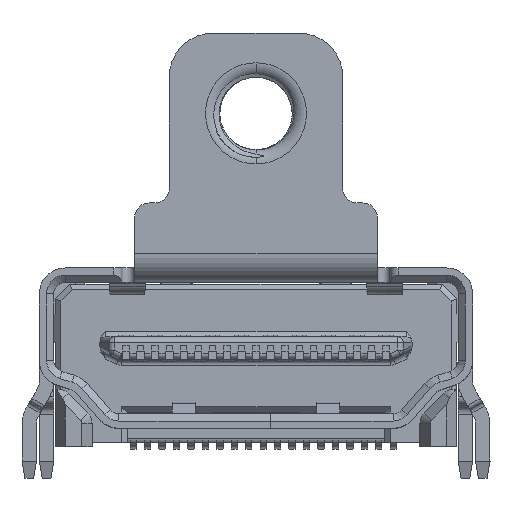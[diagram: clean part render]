
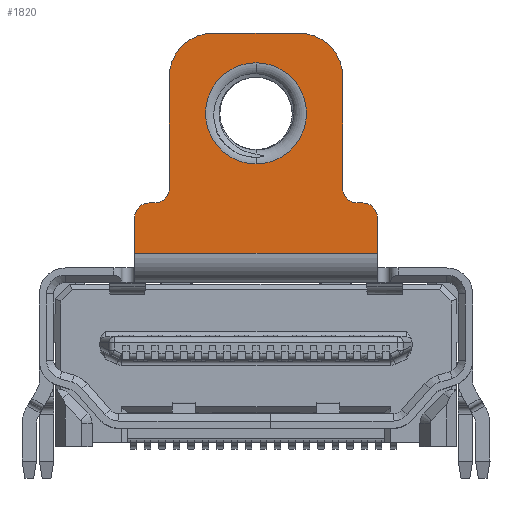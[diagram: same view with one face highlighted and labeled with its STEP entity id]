
A CAD part, top view. The second image highlights one B-rep face of the part: STEP entity #1820.
In plain terms, the highlighted face is planar.
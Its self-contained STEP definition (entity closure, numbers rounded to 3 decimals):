
#580 = VECTOR ( 'NONE', #24201, 1000. ) ;
#750 = CARTESIAN_POINT ( 'NONE',  ( 1.5, 6.8, -10.895 ) ) ;
#1609 = ORIENTED_EDGE ( 'NONE', *, *, #46197, .T. ) ;
#1820 = ADVANCED_FACE ( 'NONE', ( #32418, #22516 ), #21878, .T. ) ;
#2131 = VECTOR ( 'NONE', #45200, 1000. ) ;
#2331 = ORIENTED_EDGE ( 'NONE', *, *, #15120, .T. ) ;
#3281 = VERTEX_POINT ( 'NONE', #9397 ) ;
#3532 = VERTEX_POINT ( 'NONE', #43839 ) ;
#3802 = LINE ( 'NONE', #49220, #41613 ) ;
#4128 = DIRECTION ( 'NONE',  ( 0., 0., -1. ) ) ;
#4738 = VERTEX_POINT ( 'NONE', #27010 ) ;
#5189 = EDGE_CURVE ( 'NONE', #3281, #61666, #43744, .T. ) ;
#5857 = EDGE_CURVE ( 'NONE', #8849, #52406, #40509, .T. ) ;
#6361 = VERTEX_POINT ( 'NONE', #56551 ) ;
#6584 = CARTESIAN_POINT ( 'NONE',  ( 0., 6.8, -10.895 ) ) ;
#6742 = DIRECTION ( 'NONE',  ( 0., 0., -1. ) ) ;
#7029 = ORIENTED_EDGE ( 'NONE', *, *, #46232, .T. ) ;
#7572 = CARTESIAN_POINT ( 'NONE',  ( -3., 6.8, -5.525 ) ) ;
#7725 = CIRCLE ( 'NONE', #44523, 1.5 ) ;
#7940 = VERTEX_POINT ( 'NONE', #11384 ) ;
#8072 = CARTESIAN_POINT ( 'NONE',  ( 0., 6.8, -9.875 ) ) ;
#8609 = ORIENTED_EDGE ( 'NONE', *, *, #19757, .T. ) ;
#8689 = DIRECTION ( 'NONE',  ( 0., 0., -1. ) ) ;
#8849 = VERTEX_POINT ( 'NONE', #57715 ) ;
#9361 = ORIENTED_EDGE ( 'NONE', *, *, #19147, .T. ) ;
#9397 = CARTESIAN_POINT ( 'NONE',  ( 3.5, 6.8, -5.025 ) ) ;
#9539 = CARTESIAN_POINT ( 'NONE',  ( 3., 6.8, -5.525 ) ) ;
#10849 = LINE ( 'NONE', #29990, #25961 ) ;
#11264 = EDGE_LOOP ( 'NONE', ( #29514, #7029 ) ) ;
#11384 = CARTESIAN_POINT ( 'NONE',  ( 0., 6.8, -6.375 ) ) ;
#11802 = DIRECTION ( 'NONE',  ( 0., 1., 0. ) ) ;
#12828 = CARTESIAN_POINT ( 'NONE',  ( 0., 6.8, -8.125 ) ) ;
#13257 = VECTOR ( 'NONE', #26363, 1000. ) ;
#13549 = ORIENTED_EDGE ( 'NONE', *, *, #5189, .T. ) ;
#13586 = CARTESIAN_POINT ( 'NONE',  ( 3.7, 6.8, -5.025 ) ) ;
#14172 = AXIS2_PLACEMENT_3D ( 'NONE', #24169, #33727, #8689 ) ;
#14520 = VERTEX_POINT ( 'NONE', #63652 ) ;
#15120 = EDGE_CURVE ( 'NONE', #6361, #4738, #10849, .T. ) ;
#16145 = LINE ( 'NONE', #56657, #33399 ) ;
#16189 = EDGE_CURVE ( 'NONE', #18812, #3281, #16145, .T. ) ;
#16473 = DIRECTION ( 'NONE',  ( 0., -1., 0. ) ) ;
#17339 = CIRCLE ( 'NONE', #22622, 1.75 ) ;
#17602 = DIRECTION ( 'NONE',  ( 0., -1., 0. ) ) ;
#18812 = VERTEX_POINT ( 'NONE', #13586 ) ;
#19147 = EDGE_CURVE ( 'NONE', #33717, #3532, #30390, .T. ) ;
#19757 = EDGE_CURVE ( 'NONE', #42101, #14520, #56606, .T. ) ;
#20104 = ORIENTED_EDGE ( 'NONE', *, *, #43718, .T. ) ;
#20113 = CARTESIAN_POINT ( 'NONE',  ( 3., 6.8, -9.395 ) ) ;
#20410 = LINE ( 'NONE', #45136, #58831 ) ;
#21435 = DIRECTION ( 'NONE',  ( -1., 0., 0. ) ) ;
#21878 = PLANE ( 'NONE',  #31993 ) ;
#22148 = VERTEX_POINT ( 'NONE', #7572 ) ;
#22516 = FACE_OUTER_BOUND ( 'NONE', #31490, .T. ) ;
#22622 = AXIS2_PLACEMENT_3D ( 'NONE', #53140, #32437, #62998 ) ;
#23358 = AXIS2_PLACEMENT_3D ( 'NONE', #31317, #16473, #36590 ) ;
#24169 = CARTESIAN_POINT ( 'NONE',  ( -3.7, 6.8, -4.525 ) ) ;
#24201 = DIRECTION ( 'NONE',  ( 1., 0., 0. ) ) ;
#25704 = VERTEX_POINT ( 'NONE', #8072 ) ;
#25786 = CARTESIAN_POINT ( 'NONE',  ( 4.2, 6.8, -3.275 ) ) ;
#25961 = VECTOR ( 'NONE', #50699, 1000. ) ;
#26244 = VERTEX_POINT ( 'NONE', #29703 ) ;
#26363 = DIRECTION ( 'NONE',  ( 0., 0., 1. ) ) ;
#26428 = VECTOR ( 'NONE', #38406, 1000. ) ;
#26510 = CARTESIAN_POINT ( 'NONE',  ( -1.5, 6.8, -9.395 ) ) ;
#27010 = CARTESIAN_POINT ( 'NONE',  ( -3.7, 6.8, -5.025 ) ) ;
#27686 = ORIENTED_EDGE ( 'NONE', *, *, #51094, .T. ) ;
#28202 = EDGE_CURVE ( 'NONE', #14520, #26244, #7725, .T. ) ;
#29514 = ORIENTED_EDGE ( 'NONE', *, *, #30823, .T. ) ;
#29661 = EDGE_CURVE ( 'NONE', #4738, #33717, #34187, .T. ) ;
#29703 = CARTESIAN_POINT ( 'NONE',  ( -3., 6.8, -9.395 ) ) ;
#29990 = CARTESIAN_POINT ( 'NONE',  ( 0., 6.8, -5.025 ) ) ;
#30390 = LINE ( 'NONE', #61270, #2131 ) ;
#30676 = CIRCLE ( 'NONE', #63218, 1.5 ) ;
#30823 = EDGE_CURVE ( 'NONE', #7940, #25704, #17339, .T. ) ;
#31317 = CARTESIAN_POINT ( 'NONE',  ( -3.5, 6.8, -5.525 ) ) ;
#31490 = EDGE_LOOP ( 'NONE', ( #13549, #47265, #27686, #8609, #52278, #20104, #1609, #2331, #35665, #9361, #51469, #33424, #44672, #55272 ) ) ;
#31909 = DIRECTION ( 'NONE',  ( 0., 0., 1. ) ) ;
#31993 = AXIS2_PLACEMENT_3D ( 'NONE', #47862, #42602, #36704 ) ;
#32418 = FACE_BOUND ( 'NONE', #11264, .T. ) ;
#32437 = DIRECTION ( 'NONE',  ( 0., -1., 0. ) ) ;
#33399 = VECTOR ( 'NONE', #21435, 1000. ) ;
#33424 = ORIENTED_EDGE ( 'NONE', *, *, #5857, .F. ) ;
#33717 = VERTEX_POINT ( 'NONE', #37064 ) ;
#33727 = DIRECTION ( 'NONE',  ( 0., 1., 0. ) ) ;
#33815 = VERTEX_POINT ( 'NONE', #20113 ) ;
#34187 = CIRCLE ( 'NONE', #14172, 0.5 ) ;
#34372 = DIRECTION ( 'NONE',  ( 1., 0., 0. ) ) ;
#35090 = EDGE_CURVE ( 'NONE', #8849, #18812, #36728, .T. ) ;
#35638 = AXIS2_PLACEMENT_3D ( 'NONE', #37831, #11802, #31909 ) ;
#35665 = ORIENTED_EDGE ( 'NONE', *, *, #29661, .T. ) ;
#36590 = DIRECTION ( 'NONE',  ( 0., 0., 1. ) ) ;
#36704 = DIRECTION ( 'NONE',  ( 0., 0., 1. ) ) ;
#36728 = CIRCLE ( 'NONE', #35638, 0.5 ) ;
#37064 = CARTESIAN_POINT ( 'NONE',  ( -4.2, 6.8, -4.525 ) ) ;
#37710 = DIRECTION ( 'NONE',  ( 1., 0., 0. ) ) ;
#37831 = CARTESIAN_POINT ( 'NONE',  ( 3.7, 6.8, -4.525 ) ) ;
#38195 = DIRECTION ( 'NONE',  ( 0., 0., 1. ) ) ;
#38406 = DIRECTION ( 'NONE',  ( -1., 0., 0. ) ) ;
#40509 = LINE ( 'NONE', #51363, #13257 ) ;
#41613 = VECTOR ( 'NONE', #4128, 1000. ) ;
#42101 = VERTEX_POINT ( 'NONE', #750 ) ;
#42602 = DIRECTION ( 'NONE',  ( 0., 1., 0. ) ) ;
#43718 = EDGE_CURVE ( 'NONE', #26244, #22148, #20410, .T. ) ;
#43744 = CIRCLE ( 'NONE', #61559, 0.5 ) ;
#43839 = CARTESIAN_POINT ( 'NONE',  ( -4.2, 6.8, -3.275 ) ) ;
#44523 = AXIS2_PLACEMENT_3D ( 'NONE', #26510, #46577, #6742 ) ;
#44599 = LINE ( 'NONE', #64994, #580 ) ;
#44672 = ORIENTED_EDGE ( 'NONE', *, *, #35090, .T. ) ;
#45136 = CARTESIAN_POINT ( 'NONE',  ( -3., 6.8, -7.085 ) ) ;
#45200 = DIRECTION ( 'NONE',  ( 0., 0., 1. ) ) ;
#46197 = EDGE_CURVE ( 'NONE', #22148, #6361, #47523, .T. ) ;
#46232 = EDGE_CURVE ( 'NONE', #25704, #7940, #48594, .T. ) ;
#46577 = DIRECTION ( 'NONE',  ( 0., 1., 0. ) ) ;
#47265 = ORIENTED_EDGE ( 'NONE', *, *, #56999, .T. ) ;
#47523 = CIRCLE ( 'NONE', #23358, 0.5 ) ;
#47862 = CARTESIAN_POINT ( 'NONE',  ( -4.368, 6.8, -11.047 ) ) ;
#48594 = CIRCLE ( 'NONE', #54884, 1.75 ) ;
#49220 = CARTESIAN_POINT ( 'NONE',  ( 3., 6.8, -7.085 ) ) ;
#50699 = DIRECTION ( 'NONE',  ( -1., 0., 0. ) ) ;
#51094 = EDGE_CURVE ( 'NONE', #33815, #42101, #30676, .T. ) ;
#51363 = CARTESIAN_POINT ( 'NONE',  ( 4.2, 6.8, -3.413 ) ) ;
#51469 = ORIENTED_EDGE ( 'NONE', *, *, #57061, .T. ) ;
#52278 = ORIENTED_EDGE ( 'NONE', *, *, #28202, .T. ) ;
#52406 = VERTEX_POINT ( 'NONE', #25786 ) ;
#53140 = CARTESIAN_POINT ( 'NONE',  ( 0., 6.8, -8.125 ) ) ;
#53147 = CARTESIAN_POINT ( 'NONE',  ( 3.5, 6.8, -5.525 ) ) ;
#53473 = CARTESIAN_POINT ( 'NONE',  ( 1.5, 6.8, -9.395 ) ) ;
#53659 = DIRECTION ( 'NONE',  ( 0., -1., 0. ) ) ;
#54440 = DIRECTION ( 'NONE',  ( 0., 1., 0. ) ) ;
#54884 = AXIS2_PLACEMENT_3D ( 'NONE', #12828, #53659, #38195 ) ;
#55272 = ORIENTED_EDGE ( 'NONE', *, *, #16189, .T. ) ;
#56551 = CARTESIAN_POINT ( 'NONE',  ( -3.5, 6.8, -5.025 ) ) ;
#56606 = LINE ( 'NONE', #6584, #26428 ) ;
#56657 = CARTESIAN_POINT ( 'NONE',  ( 0., 6.8, -5.025 ) ) ;
#56999 = EDGE_CURVE ( 'NONE', #61666, #33815, #3802, .T. ) ;
#57061 = EDGE_CURVE ( 'NONE', #3532, #52406, #44599, .T. ) ;
#57715 = CARTESIAN_POINT ( 'NONE',  ( 4.2, 6.8, -4.525 ) ) ;
#58831 = VECTOR ( 'NONE', #60567, 1000. ) ;
#60567 = DIRECTION ( 'NONE',  ( 0., 0., 1. ) ) ;
#61270 = CARTESIAN_POINT ( 'NONE',  ( -4.2, 6.8, -3.413 ) ) ;
#61559 = AXIS2_PLACEMENT_3D ( 'NONE', #53147, #17602, #37710 ) ;
#61666 = VERTEX_POINT ( 'NONE', #9539 ) ;
#62998 = DIRECTION ( 'NONE',  ( 0., 0., 1. ) ) ;
#63218 = AXIS2_PLACEMENT_3D ( 'NONE', #53473, #54440, #34372 ) ;
#63652 = CARTESIAN_POINT ( 'NONE',  ( -1.5, 6.8, -10.895 ) ) ;
#64994 = CARTESIAN_POINT ( 'NONE',  ( 0., 6.8, -3.275 ) ) ;
